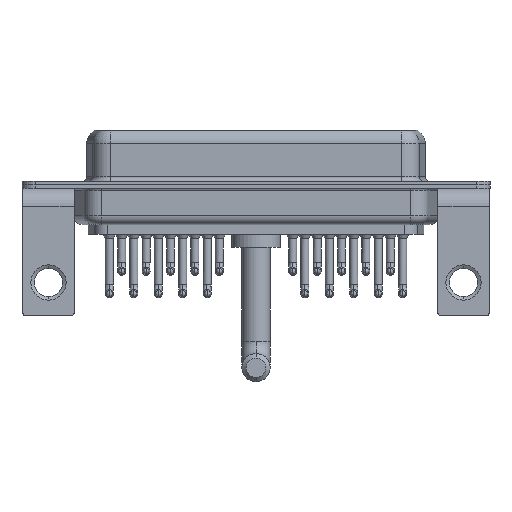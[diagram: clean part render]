
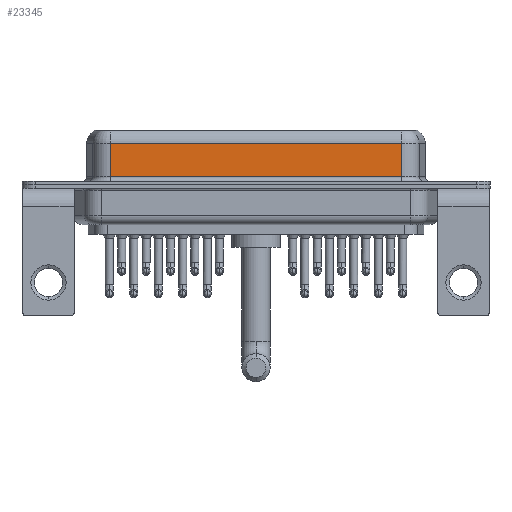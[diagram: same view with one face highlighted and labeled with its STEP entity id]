
A CAD part, front view. The second image highlights one B-rep face of the part: STEP entity #23345.
In plain terms, the highlighted planar face has unit normal (0, -1, 0).
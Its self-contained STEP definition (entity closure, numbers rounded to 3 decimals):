
#2730 = LINE ( 'NONE', #18928, #11052 ) ;
#2809 = VERTEX_POINT ( 'NONE', #11054 ) ;
#2985 = ORIENTED_EDGE ( 'NONE', *, *, #13084, .T. ) ;
#3677 = DIRECTION ( 'NONE',  ( 0., 0., 1. ) ) ;
#4628 = VERTEX_POINT ( 'NONE', #10561 ) ;
#5858 = VECTOR ( 'NONE', #11192, 1000. ) ;
#5902 = CARTESIAN_POINT ( 'NONE',  ( 40.037, -3.95, 4.65 ) ) ;
#7705 = DIRECTION ( 'NONE',  ( 0., 0., -1. ) ) ;
#8083 = LINE ( 'NONE', #11658, #14592 ) ;
#8257 = ORIENTED_EDGE ( 'NONE', *, *, #13820, .T. ) ;
#8611 = ORIENTED_EDGE ( 'NONE', *, *, #11846, .F. ) ;
#9117 = ORIENTED_EDGE ( 'NONE', *, *, #21721, .T. ) ;
#9870 = DIRECTION ( 'NONE',  ( 0., 0., -1. ) ) ;
#9942 = CARTESIAN_POINT ( 'NONE',  ( 40.037, -3.95, 0.9 ) ) ;
#10017 = VERTEX_POINT ( 'NONE', #16242 ) ;
#10561 = CARTESIAN_POINT ( 'NONE',  ( 40.037, -3.95, 4.65 ) ) ;
#10998 = VERTEX_POINT ( 'NONE', #9942 ) ;
#11052 = VECTOR ( 'NONE', #7705, 1000. ) ;
#11054 = CARTESIAN_POINT ( 'NONE',  ( 7.013, -3.95, 4.65 ) ) ;
#11192 = DIRECTION ( 'NONE',  ( 1., 0., 0. ) ) ;
#11658 = CARTESIAN_POINT ( 'NONE',  ( 40.037, -3.95, 6.4 ) ) ;
#11846 = EDGE_CURVE ( 'NONE', #4628, #10998, #8083, .T. ) ;
#12667 = FACE_OUTER_BOUND ( 'NONE', #14015, .T. ) ;
#12962 = LINE ( 'NONE', #20172, #5858 ) ;
#13084 = EDGE_CURVE ( 'NONE', #10017, #10998, #12962, .T. ) ;
#13749 = AXIS2_PLACEMENT_3D ( 'NONE', #20000, #22015, #3677 ) ;
#13820 = EDGE_CURVE ( 'NONE', #4628, #2809, #17757, .T. ) ;
#14015 = EDGE_LOOP ( 'NONE', ( #8611, #8257, #9117, #2985 ) ) ;
#14592 = VECTOR ( 'NONE', #9870, 1000. ) ;
#16242 = CARTESIAN_POINT ( 'NONE',  ( 7.013, -3.95, 0.9 ) ) ;
#16570 = DIRECTION ( 'NONE',  ( -1., 0., 0. ) ) ;
#17354 = VECTOR ( 'NONE', #16570, 1000. ) ;
#17757 = LINE ( 'NONE', #5902, #17354 ) ;
#18342 = PLANE ( 'NONE',  #13749 ) ;
#18928 = CARTESIAN_POINT ( 'NONE',  ( 7.013, -3.95, 6.4 ) ) ;
#20000 = CARTESIAN_POINT ( 'NONE',  ( 40.037, -3.95, 6.4 ) ) ;
#20172 = CARTESIAN_POINT ( 'NONE',  ( 40.037, -3.95, 0.9 ) ) ;
#21721 = EDGE_CURVE ( 'NONE', #2809, #10017, #2730, .T. ) ;
#22015 = DIRECTION ( 'NONE',  ( 0., 1., 0. ) ) ;
#23345 = ADVANCED_FACE ( 'NONE', ( #12667 ), #18342, .F. ) ;
